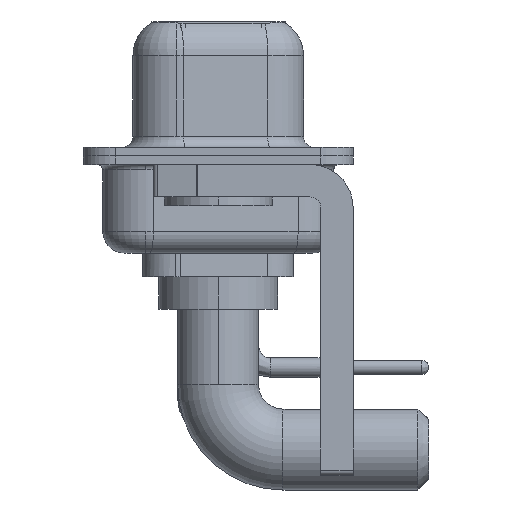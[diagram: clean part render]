
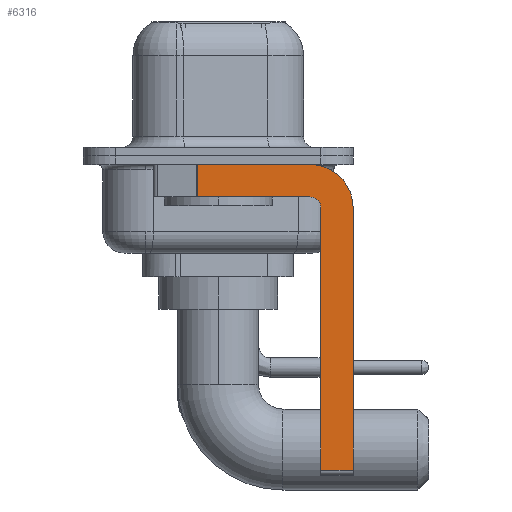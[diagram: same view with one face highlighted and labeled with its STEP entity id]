
A CAD part, left-side view. The second image highlights one B-rep face of the part: STEP entity #6316.
In plain terms, the highlighted planar face has unit normal (-1, 0, 0).
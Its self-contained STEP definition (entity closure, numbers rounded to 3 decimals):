
#166 = LINE ( 'NONE', #22066, #24311 ) ;
#479 = ORIENTED_EDGE ( 'NONE', *, *, #12815, .F. ) ;
#1413 = AXIS2_PLACEMENT_3D ( 'NONE', #18763, #18885, #24951 ) ;
#1818 = LINE ( 'NONE', #18108, #14307 ) ;
#1864 = DIRECTION ( 'NONE',  ( 0., 0., -1. ) ) ;
#2075 = DIRECTION ( 'NONE',  ( 0., 1., 0. ) ) ;
#2278 = CARTESIAN_POINT ( 'NONE',  ( -2.9, -6.25, -2.4 ) ) ;
#2321 = LINE ( 'NONE', #16192, #16845 ) ;
#2323 = CARTESIAN_POINT ( 'NONE',  ( -2.9, -4.75, -14.55 ) ) ;
#2382 = DIRECTION ( 'NONE',  ( 1., 0., 0. ) ) ;
#3593 = DIRECTION ( 'NONE',  ( 0., -1., 0. ) ) ;
#4722 = CIRCLE ( 'NONE', #1413, 0.5 ) ;
#5504 = ORIENTED_EDGE ( 'NONE', *, *, #13737, .T. ) ;
#5526 = VERTEX_POINT ( 'NONE', #9709 ) ;
#5585 = CIRCLE ( 'NONE', #18817, 2. ) ;
#5658 = VECTOR ( 'NONE', #18875, 1000. ) ;
#5742 = PLANE ( 'NONE',  #8618 ) ;
#5780 = EDGE_CURVE ( 'NONE', #6060, #18397, #14872, .T. ) ;
#5876 = FACE_OUTER_BOUND ( 'NONE', #14638, .T. ) ;
#6060 = VERTEX_POINT ( 'NONE', #2278 ) ;
#6136 = CARTESIAN_POINT ( 'NONE',  ( -2.9, -4.25, -2.4 ) ) ;
#6316 = ADVANCED_FACE ( 'NONE', ( #5876 ), #5742, .F. ) ;
#6389 = CARTESIAN_POINT ( 'NONE',  ( -2.9, 0.978, -0.4 ) ) ;
#6689 = CARTESIAN_POINT ( 'NONE',  ( -2.9, -6.25, -14.55 ) ) ;
#6911 = ORIENTED_EDGE ( 'NONE', *, *, #12019, .F. ) ;
#8618 = AXIS2_PLACEMENT_3D ( 'NONE', #6136, #19865, #1864 ) ;
#9250 = CARTESIAN_POINT ( 'NONE',  ( -2.9, 0.978, -1.9 ) ) ;
#9273 = EDGE_CURVE ( 'NONE', #5526, #19101, #2321, .T. ) ;
#9327 = LINE ( 'NONE', #13857, #17128 ) ;
#9709 = CARTESIAN_POINT ( 'NONE',  ( -2.9, -4.25, -1.9 ) ) ;
#10023 = EDGE_CURVE ( 'NONE', #11515, #16151, #21352, .T. ) ;
#10271 = CARTESIAN_POINT ( 'NONE',  ( -2.9, -4.25, -2.4 ) ) ;
#11515 = VERTEX_POINT ( 'NONE', #6389 ) ;
#11863 = EDGE_CURVE ( 'NONE', #11515, #19101, #9327, .T. ) ;
#12019 = EDGE_CURVE ( 'NONE', #20966, #5526, #4722, .T. ) ;
#12200 = DIRECTION ( 'NONE',  ( 0., 0., 1. ) ) ;
#12413 = ORIENTED_EDGE ( 'NONE', *, *, #11863, .T. ) ;
#12702 = CARTESIAN_POINT ( 'NONE',  ( -2.9, -4.25, -0.4 ) ) ;
#12815 = EDGE_CURVE ( 'NONE', #16151, #6060, #5585, .T. ) ;
#12962 = VECTOR ( 'NONE', #3593, 1000. ) ;
#13737 = EDGE_CURVE ( 'NONE', #23123, #18397, #1818, .T. ) ;
#13857 = CARTESIAN_POINT ( 'NONE',  ( -2.9, 0.978, -1.9 ) ) ;
#14095 = ORIENTED_EDGE ( 'NONE', *, *, #10023, .F. ) ;
#14304 = DIRECTION ( 'NONE',  ( 0., 0., -1. ) ) ;
#14307 = VECTOR ( 'NONE', #23564, 1000. ) ;
#14638 = EDGE_LOOP ( 'NONE', ( #14095, #12413, #23740, #6911, #23604, #5504, #19519, #479 ) ) ;
#14872 = LINE ( 'NONE', #22761, #5658 ) ;
#16151 = VERTEX_POINT ( 'NONE', #12702 ) ;
#16192 = CARTESIAN_POINT ( 'NONE',  ( -2.9, -4.25, -1.9 ) ) ;
#16845 = VECTOR ( 'NONE', #2075, 1000. ) ;
#17128 = VECTOR ( 'NONE', #20890, 1000. ) ;
#18108 = CARTESIAN_POINT ( 'NONE',  ( -2.9, -4.25, -14.55 ) ) ;
#18397 = VERTEX_POINT ( 'NONE', #6689 ) ;
#18763 = CARTESIAN_POINT ( 'NONE',  ( -2.9, -4.25, -2.4 ) ) ;
#18817 = AXIS2_PLACEMENT_3D ( 'NONE', #10271, #2382, #14304 ) ;
#18875 = DIRECTION ( 'NONE',  ( 0., 0., -1. ) ) ;
#18885 = DIRECTION ( 'NONE',  ( -1., 0., 0. ) ) ;
#19101 = VERTEX_POINT ( 'NONE', #9250 ) ;
#19268 = CARTESIAN_POINT ( 'NONE',  ( -2.9, 3., -0.4 ) ) ;
#19369 = CARTESIAN_POINT ( 'NONE',  ( -2.9, -4.75, -2.4 ) ) ;
#19519 = ORIENTED_EDGE ( 'NONE', *, *, #5780, .F. ) ;
#19865 = DIRECTION ( 'NONE',  ( 1., 0., 0. ) ) ;
#20890 = DIRECTION ( 'NONE',  ( 0., 0., -1. ) ) ;
#20966 = VERTEX_POINT ( 'NONE', #19369 ) ;
#21352 = LINE ( 'NONE', #19268, #12962 ) ;
#22066 = CARTESIAN_POINT ( 'NONE',  ( -2.9, -4.75, -14.8 ) ) ;
#22761 = CARTESIAN_POINT ( 'NONE',  ( -2.9, -6.25, -2.4 ) ) ;
#23123 = VERTEX_POINT ( 'NONE', #2323 ) ;
#23564 = DIRECTION ( 'NONE',  ( 0., -1., 0. ) ) ;
#23604 = ORIENTED_EDGE ( 'NONE', *, *, #23616, .F. ) ;
#23616 = EDGE_CURVE ( 'NONE', #23123, #20966, #166, .T. ) ;
#23740 = ORIENTED_EDGE ( 'NONE', *, *, #9273, .F. ) ;
#24311 = VECTOR ( 'NONE', #12200, 1000. ) ;
#24951 = DIRECTION ( 'NONE',  ( 0., 0., 1. ) ) ;
